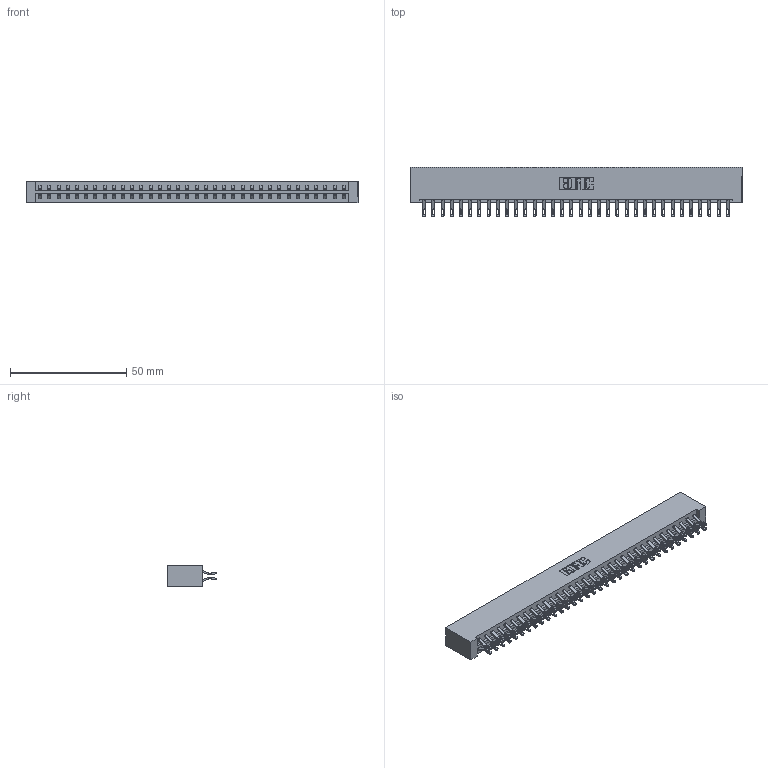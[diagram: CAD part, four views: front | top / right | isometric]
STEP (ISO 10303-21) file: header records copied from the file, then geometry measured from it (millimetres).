
FILE_DESCRIPTION (( 'STEP AP203' ), '1' );
FILE_NAME ('833-068-555-201.STEP', '2020-06-05T11:02:47', ( '' ), ( '' ), 'SwSTEP 2.0', 'SolidWorks 2020', '' );
FILE_SCHEMA (( 'CONFIG_CONTROL_DESIGN' ));
Length unit declared in the file: inch
Products named in the file (3): 833 Part_Lugless; 345-292-001_555 Tail; 833-068-555-201
Assembly tree (69 placements, depth 2):
  833-068-555-201
    833 Part_Lugless
    345-292-001_555 Tail  x68
Bounding box: 142.98 x 21.47 x 9.4 mm (x, y, z)
Volume: 15351.7 mm3; surface area: 18825.6 mm2
Topology: 69 solids, 69 shells, 4050 faces, 12731 edges, 8486 vertices
Faces by surface type: plane 2378, cylinder 1672
Entity records: 22957 total; most frequent: CARTESIAN_POINT 3848, ORIENTED_EDGE 3754, DIRECTION 3265, EDGE_CURVE 1877, VECTOR 1737, LINE 1737, VERTEX_POINT 1250, AXIS2_PLACEMENT_3D 764
